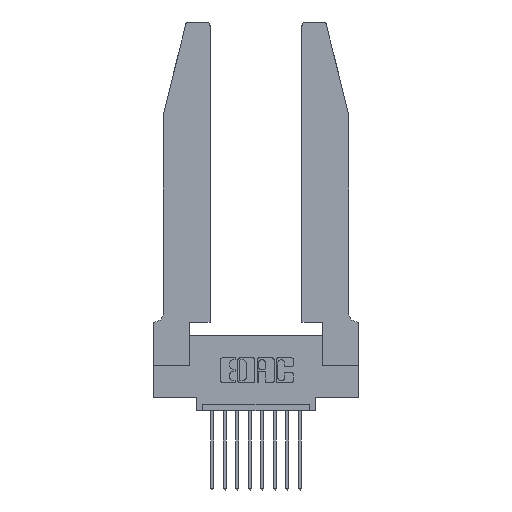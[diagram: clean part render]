
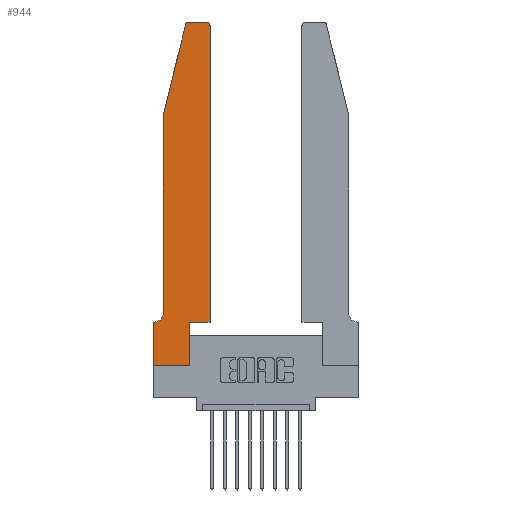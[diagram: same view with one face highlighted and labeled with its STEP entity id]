
A CAD part, top view. The second image highlights one B-rep face of the part: STEP entity #944.
In plain terms, the highlighted planar face has unit normal (0, 0, 1).
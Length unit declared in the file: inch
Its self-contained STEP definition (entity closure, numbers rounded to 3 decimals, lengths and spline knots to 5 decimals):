
#122 = CARTESIAN_POINT ( 'NONE',  ( 0.284, 2.75, 0.37 ) ) ;
#229 = CARTESIAN_POINT ( 'NONE',  ( 0.4505, 2.72, 0.37 ) ) ;
#263 = DIRECTION ( 'NONE',  ( -1., 0., 0. ) ) ;
#400 = VERTEX_POINT ( 'NONE', #3659 ) ;
#615 = VECTOR ( 'NONE', #8504, 39.37008 ) ;
#716 = ORIENTED_EDGE ( 'NONE', *, *, #4098, .T. ) ;
#907 = EDGE_CURVE ( 'NONE', #2896, #976, #4043, .T. ) ;
#931 = CARTESIAN_POINT ( 'NONE',  ( 0.0755, 0.42, 0.37 ) ) ;
#944 = ADVANCED_FACE ( 'NONE', ( #3867 ), #12491, .T. ) ;
#976 = VERTEX_POINT ( 'NONE', #931 ) ;
#1084 = EDGE_CURVE ( 'NONE', #12251, #11041, #5541, .T. ) ;
#1544 = DIRECTION ( 'NONE',  ( 1., 0., 0. ) ) ;
#1724 = AXIS2_PLACEMENT_3D ( 'NONE', #12566, #6553, #7853 ) ;
#1731 = CARTESIAN_POINT ( 'NONE',  ( 0.0755, 2., 0.37 ) ) ;
#1978 = DIRECTION ( 'NONE',  ( 1., 0., 0. ) ) ;
#2286 = ORIENTED_EDGE ( 'NONE', *, *, #1084, .T. ) ;
#2399 = EDGE_CURVE ( 'NONE', #14461, #3618, #8292, .T. ) ;
#2673 = CARTESIAN_POINT ( 'NONE',  ( 0., 0.35, 0.37 ) ) ;
#2752 = EDGE_CURVE ( 'NONE', #6495, #12251, #12644, .T. ) ;
#2896 = VERTEX_POINT ( 'NONE', #12053 ) ;
#3182 = CARTESIAN_POINT ( 'NONE',  ( 0.2605, 2.75, 0.37 ) ) ;
#3252 = DIRECTION ( 'NONE',  ( 1., 0., 0. ) ) ;
#3321 = VECTOR ( 'NONE', #3663, 39.37008 ) ;
#3491 = LINE ( 'NONE', #13727, #13628 ) ;
#3618 = VERTEX_POINT ( 'NONE', #7944 ) ;
#3659 = CARTESIAN_POINT ( 'NONE',  ( 0.4205, 2.75, 0.37 ) ) ;
#3663 = DIRECTION ( 'NONE',  ( 0., -1., 0. ) ) ;
#3666 = AXIS2_PLACEMENT_3D ( 'NONE', #13325, #11122, #1544 ) ;
#3831 = VERTEX_POINT ( 'NONE', #11024 ) ;
#3867 = FACE_OUTER_BOUND ( 'NONE', #13103, .T. ) ;
#3931 = CARTESIAN_POINT ( 'NONE',  ( 0.0055, 0.35, 0.37 ) ) ;
#4043 = LINE ( 'NONE', #1731, #12894 ) ;
#4049 = CARTESIAN_POINT ( 'NONE',  ( 0.2865, 0., 0.37 ) ) ;
#4098 = EDGE_CURVE ( 'NONE', #14005, #7470, #10904, .T. ) ;
#4355 = EDGE_CURVE ( 'NONE', #3618, #2896, #9374, .T. ) ;
#5050 = CARTESIAN_POINT ( 'NONE',  ( 0., 0., 0.37 ) ) ;
#5541 = LINE ( 'NONE', #5050, #3321 ) ;
#5574 = ORIENTED_EDGE ( 'NONE', *, *, #6737, .T. ) ;
#5688 = ORIENTED_EDGE ( 'NONE', *, *, #2399, .T. ) ;
#6163 = VECTOR ( 'NONE', #13298, 39.37008 ) ;
#6495 = VERTEX_POINT ( 'NONE', #3931 ) ;
#6553 = DIRECTION ( 'NONE',  ( 0., 0., 1. ) ) ;
#6644 = LINE ( 'NONE', #12721, #11760 ) ;
#6645 = EDGE_CURVE ( 'NONE', #11041, #10693, #7022, .T. ) ;
#6737 = EDGE_CURVE ( 'NONE', #7470, #400, #14010, .T. ) ;
#7022 = LINE ( 'NONE', #15115, #13834 ) ;
#7300 = CARTESIAN_POINT ( 'NONE',  ( 0.4505, 0.35, 0.37 ) ) ;
#7470 = VERTEX_POINT ( 'NONE', #229 ) ;
#7725 = VECTOR ( 'NONE', #11528, 39.37008 ) ;
#7806 = ORIENTED_EDGE ( 'NONE', *, *, #6645, .T. ) ;
#7853 = DIRECTION ( 'NONE',  ( 1., 0., 0. ) ) ;
#7944 = CARTESIAN_POINT ( 'NONE',  ( 0.25487, 2.72718, 0.37 ) ) ;
#8069 = CARTESIAN_POINT ( 'NONE',  ( 0., 0.35, 0.37 ) ) ;
#8292 = CIRCLE ( 'NONE', #3666, 0.03 ) ;
#8504 = DIRECTION ( 'NONE',  ( 0., 1., 0. ) ) ;
#8609 = VECTOR ( 'NONE', #12775, 39.37008 ) ;
#8911 = DIRECTION ( 'NONE',  ( 0., 1., 0. ) ) ;
#8995 = AXIS2_PLACEMENT_3D ( 'NONE', #12205, #13414, #263 ) ;
#9374 = LINE ( 'NONE', #13359, #6163 ) ;
#9392 = ORIENTED_EDGE ( 'NONE', *, *, #10933, .T. ) ;
#9674 = AXIS2_PLACEMENT_3D ( 'NONE', #8069, #12954, #3252 ) ;
#9706 = ORIENTED_EDGE ( 'NONE', *, *, #12196, .T. ) ;
#10693 = VERTEX_POINT ( 'NONE', #4049 ) ;
#10904 = LINE ( 'NONE', #7300, #615 ) ;
#10933 = EDGE_CURVE ( 'NONE', #400, #14461, #13908, .T. ) ;
#11024 = CARTESIAN_POINT ( 'NONE',  ( 0.2865, 0.35, 0.37 ) ) ;
#11041 = VERTEX_POINT ( 'NONE', #13126 ) ;
#11106 = ORIENTED_EDGE ( 'NONE', *, *, #4355, .T. ) ;
#11122 = DIRECTION ( 'NONE',  ( 0., 0., 1. ) ) ;
#11501 = DIRECTION ( 'NONE',  ( 0., -1., 0. ) ) ;
#11528 = DIRECTION ( 'NONE',  ( -1., 0., 0. ) ) ;
#11760 = VECTOR ( 'NONE', #1978, 39.37008 ) ;
#11982 = CIRCLE ( 'NONE', #8995, 0.07 ) ;
#12053 = CARTESIAN_POINT ( 'NONE',  ( 0.0755, 2., 0.37 ) ) ;
#12062 = DIRECTION ( 'NONE',  ( 1., 0., 0. ) ) ;
#12196 = EDGE_CURVE ( 'NONE', #976, #6495, #11982, .T. ) ;
#12205 = CARTESIAN_POINT ( 'NONE',  ( 0.0055, 0.42, 0.37 ) ) ;
#12251 = VERTEX_POINT ( 'NONE', #2673 ) ;
#12491 = PLANE ( 'NONE',  #9674 ) ;
#12566 = CARTESIAN_POINT ( 'NONE',  ( 0.4205, 2.72, 0.37 ) ) ;
#12640 = CARTESIAN_POINT ( 'NONE',  ( 0.0755, 0.35, 0.37 ) ) ;
#12644 = LINE ( 'NONE', #12640, #7725 ) ;
#12721 = CARTESIAN_POINT ( 'NONE',  ( 0.4505, 0.35, 0.37 ) ) ;
#12775 = DIRECTION ( 'NONE',  ( -1., 0., 0. ) ) ;
#12894 = VECTOR ( 'NONE', #11501, 39.37008 ) ;
#12954 = DIRECTION ( 'NONE',  ( 0., 0., 1. ) ) ;
#13103 = EDGE_LOOP ( 'NONE', ( #9392, #5688, #11106, #14529, #9706, #13741, #2286, #7806, #15426, #13573, #716, #5574 ) ) ;
#13126 = CARTESIAN_POINT ( 'NONE',  ( 0., 0., 0.37 ) ) ;
#13298 = DIRECTION ( 'NONE',  ( -0.239, -0.971, 0. ) ) ;
#13325 = CARTESIAN_POINT ( 'NONE',  ( 0.284, 2.72, 0.37 ) ) ;
#13359 = CARTESIAN_POINT ( 'NONE',  ( 0.0755, 2., 0.37 ) ) ;
#13392 = CARTESIAN_POINT ( 'NONE',  ( 0.4505, 0.35, 0.37 ) ) ;
#13414 = DIRECTION ( 'NONE',  ( 0., 0., -1. ) ) ;
#13483 = EDGE_CURVE ( 'NONE', #10693, #3831, #3491, .T. ) ;
#13573 = ORIENTED_EDGE ( 'NONE', *, *, #13582, .T. ) ;
#13582 = EDGE_CURVE ( 'NONE', #3831, #14005, #6644, .T. ) ;
#13628 = VECTOR ( 'NONE', #8911, 39.37008 ) ;
#13727 = CARTESIAN_POINT ( 'NONE',  ( 0.2865, 0.35, 0.37 ) ) ;
#13741 = ORIENTED_EDGE ( 'NONE', *, *, #2752, .T. ) ;
#13834 = VECTOR ( 'NONE', #12062, 39.37008 ) ;
#13908 = LINE ( 'NONE', #3182, #8609 ) ;
#14005 = VERTEX_POINT ( 'NONE', #13392 ) ;
#14010 = CIRCLE ( 'NONE', #1724, 0.03 ) ;
#14461 = VERTEX_POINT ( 'NONE', #122 ) ;
#14529 = ORIENTED_EDGE ( 'NONE', *, *, #907, .T. ) ;
#15115 = CARTESIAN_POINT ( 'NONE',  ( 0., 0., 0.37 ) ) ;
#15426 = ORIENTED_EDGE ( 'NONE', *, *, #13483, .T. ) ;
